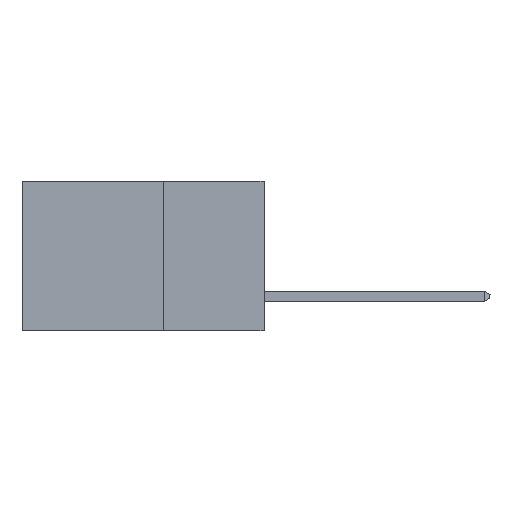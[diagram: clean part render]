
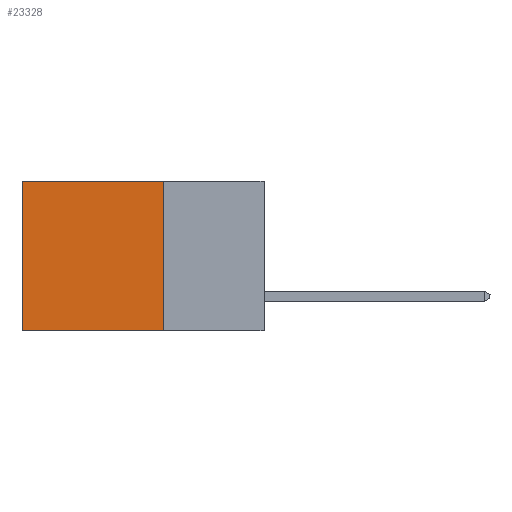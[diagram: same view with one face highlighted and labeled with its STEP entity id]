
A CAD part, left-side view. The second image highlights one B-rep face of the part: STEP entity #23328.
In plain terms, the highlighted planar face has unit normal (-1, 0, 0).
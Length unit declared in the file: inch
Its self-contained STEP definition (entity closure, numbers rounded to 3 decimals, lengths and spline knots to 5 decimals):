
#1045 = DIRECTION ( 'NONE',  ( 0., 0., -1. ) ) ;
#1348 = CARTESIAN_POINT ( 'NONE',  ( 0.298, 0.6, 0. ) ) ;
#1392 = VERTEX_POINT ( 'NONE', #11406 ) ;
#1469 = ORIENTED_EDGE ( 'NONE', *, *, #21361, .F. ) ;
#1712 = ORIENTED_EDGE ( 'NONE', *, *, #25617, .T. ) ;
#2816 = CARTESIAN_POINT ( 'NONE',  ( 0.298, 0.25, 0. ) ) ;
#2876 = DIRECTION ( 'NONE',  ( 0., 1., 0. ) ) ;
#3620 = LINE ( 'NONE', #31144, #23693 ) ;
#5465 = CARTESIAN_POINT ( 'NONE',  ( 0.298, 0.25, -0.37 ) ) ;
#6218 = LINE ( 'NONE', #5465, #21283 ) ;
#6765 = DIRECTION ( 'NONE',  ( 1., 0., 0. ) ) ;
#7304 = VERTEX_POINT ( 'NONE', #23642 ) ;
#8767 = AXIS2_PLACEMENT_3D ( 'NONE', #21559, #6765, #9381 ) ;
#9381 = DIRECTION ( 'NONE',  ( 0., 0., -1. ) ) ;
#10659 = LINE ( 'NONE', #2816, #13280 ) ;
#10736 = CARTESIAN_POINT ( 'NONE',  ( 0.298, 0.6, 0. ) ) ;
#11406 = CARTESIAN_POINT ( 'NONE',  ( 0.298, 0.25, 0. ) ) ;
#12658 = VERTEX_POINT ( 'NONE', #10736 ) ;
#13280 = VECTOR ( 'NONE', #14913, 39.37008 ) ;
#14377 = ORIENTED_EDGE ( 'NONE', *, *, #14512, .T. ) ;
#14512 = EDGE_CURVE ( 'NONE', #12658, #7304, #25377, .T. ) ;
#14913 = DIRECTION ( 'NONE',  ( 0., 0., -1. ) ) ;
#15738 = VECTOR ( 'NONE', #1045, 39.37008 ) ;
#16362 = ORIENTED_EDGE ( 'NONE', *, *, #27005, .F. ) ;
#16497 = PLANE ( 'NONE',  #8767 ) ;
#17940 = VERTEX_POINT ( 'NONE', #29017 ) ;
#21283 = VECTOR ( 'NONE', #2876, 39.37008 ) ;
#21361 = EDGE_CURVE ( 'NONE', #17940, #7304, #6218, .T. ) ;
#21559 = CARTESIAN_POINT ( 'NONE',  ( 0.298, 0.25, 0. ) ) ;
#22700 = FACE_OUTER_BOUND ( 'NONE', #31154, .T. ) ;
#23328 = ADVANCED_FACE ( 'NONE', ( #22700 ), #16497, .F. ) ;
#23642 = CARTESIAN_POINT ( 'NONE',  ( 0.298, 0.6, -0.37 ) ) ;
#23693 = VECTOR ( 'NONE', #26244, 39.37008 ) ;
#25377 = LINE ( 'NONE', #1348, #15738 ) ;
#25617 = EDGE_CURVE ( 'NONE', #1392, #12658, #3620, .T. ) ;
#26244 = DIRECTION ( 'NONE',  ( 0., 1., 0. ) ) ;
#27005 = EDGE_CURVE ( 'NONE', #1392, #17940, #10659, .T. ) ;
#29017 = CARTESIAN_POINT ( 'NONE',  ( 0.298, 0.25, -0.37 ) ) ;
#31144 = CARTESIAN_POINT ( 'NONE',  ( 0.298, 0.25, 0. ) ) ;
#31154 = EDGE_LOOP ( 'NONE', ( #14377, #1469, #16362, #1712 ) ) ;
